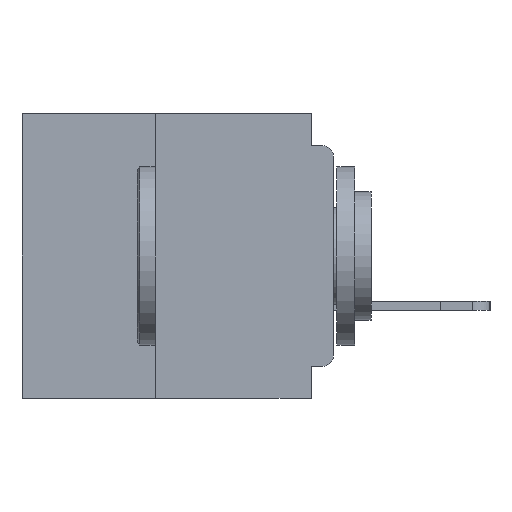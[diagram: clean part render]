
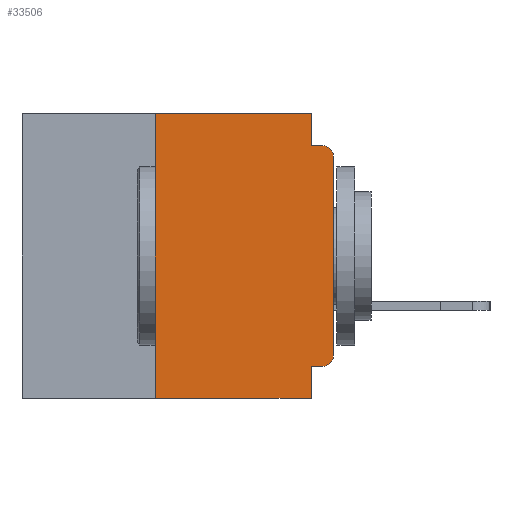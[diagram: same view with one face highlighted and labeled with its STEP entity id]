
A CAD part, left-side view. The second image highlights one B-rep face of the part: STEP entity #33506.
In plain terms, the highlighted planar face has unit normal (-1, 0, 0).
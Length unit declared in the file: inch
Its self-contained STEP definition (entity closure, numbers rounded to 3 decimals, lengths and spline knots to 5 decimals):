
#89 = LINE ( 'NONE', #6230, #43889 ) ;
#749 = EDGE_CURVE ( 'NONE', #41392, #6359, #35364, .T. ) ;
#1302 = VERTEX_POINT ( 'NONE', #23947 ) ;
#1709 = AXIS2_PLACEMENT_3D ( 'NONE', #22011, #51377, #26247 ) ;
#2447 = VECTOR ( 'NONE', #11956, 39.37008 ) ;
#2738 = VECTOR ( 'NONE', #22655, 39.37008 ) ;
#3808 = LINE ( 'NONE', #45752, #2447 ) ;
#4059 = EDGE_CURVE ( 'NONE', #29082, #25901, #21482, .T. ) ;
#4437 = VERTEX_POINT ( 'NONE', #18731 ) ;
#4647 = DIRECTION ( 'NONE',  ( 0., -1., 0. ) ) ;
#5487 = CARTESIAN_POINT ( 'NONE',  ( 0., 0.031, 0. ) ) ;
#6230 = CARTESIAN_POINT ( 'NONE',  ( 0., 0., 0. ) ) ;
#6359 = VERTEX_POINT ( 'NONE', #53056 ) ;
#6812 = LINE ( 'NONE', #17221, #50294 ) ;
#6839 = VERTEX_POINT ( 'NONE', #39576 ) ;
#7388 = DIRECTION ( 'NONE',  ( -1., 0., 0. ) ) ;
#7418 = CARTESIAN_POINT ( 'NONE',  ( 0., 0.015, -0.355 ) ) ;
#7684 = VECTOR ( 'NONE', #35061, 39.37008 ) ;
#9363 = EDGE_CURVE ( 'NONE', #1302, #6359, #6812, .T. ) ;
#10701 = PLANE ( 'NONE',  #41313 ) ;
#11185 = CARTESIAN_POINT ( 'NONE',  ( 0., 0.031, -0.045 ) ) ;
#11956 = DIRECTION ( 'NONE',  ( 0., 1., 0. ) ) ;
#12181 = EDGE_CURVE ( 'NONE', #1302, #47097, #12476, .T. ) ;
#12476 = LINE ( 'NONE', #26227, #33668 ) ;
#12588 = EDGE_CURVE ( 'NONE', #29139, #41392, #3808, .T. ) ;
#12941 = AXIS2_PLACEMENT_3D ( 'NONE', #32714, #7388, #36957 ) ;
#13385 = ORIENTED_EDGE ( 'NONE', *, *, #20022, .T. ) ;
#13660 = LINE ( 'NONE', #45556, #26240 ) ;
#14513 = EDGE_CURVE ( 'NONE', #47097, #6839, #25292, .T. ) ;
#14575 = ORIENTED_EDGE ( 'NONE', *, *, #17854, .F. ) ;
#14943 = CARTESIAN_POINT ( 'NONE',  ( 0., 0.031, -0.4 ) ) ;
#15524 = CARTESIAN_POINT ( 'NONE',  ( 0., 0., -0.06 ) ) ;
#16011 = DIRECTION ( 'NONE',  ( 0., -1., 0. ) ) ;
#17221 = CARTESIAN_POINT ( 'NONE',  ( 0., 0.437, -0.4 ) ) ;
#17854 = EDGE_CURVE ( 'NONE', #6839, #24249, #42747, .T. ) ;
#18723 = CARTESIAN_POINT ( 'NONE',  ( 0., 0.25, 0. ) ) ;
#18731 = CARTESIAN_POINT ( 'NONE',  ( 0., 0., -0.34 ) ) ;
#19205 = DIRECTION ( 'NONE',  ( 0., 0., -1. ) ) ;
#20022 = EDGE_CURVE ( 'NONE', #4437, #29082, #89, .T. ) ;
#21482 = CIRCLE ( 'NONE', #12941, 0.015 ) ;
#22011 = CARTESIAN_POINT ( 'NONE',  ( 0., 0.015, -0.34 ) ) ;
#22655 = DIRECTION ( 'NONE',  ( 0., -1., 0. ) ) ;
#23947 = CARTESIAN_POINT ( 'NONE',  ( 0., 0.25, -0.4 ) ) ;
#24110 = VECTOR ( 'NONE', #31407, 39.37008 ) ;
#24249 = VERTEX_POINT ( 'NONE', #11185 ) ;
#25292 = LINE ( 'NONE', #47868, #2738 ) ;
#25406 = ORIENTED_EDGE ( 'NONE', *, *, #12181, .F. ) ;
#25901 = VERTEX_POINT ( 'NONE', #27492 ) ;
#25913 = ORIENTED_EDGE ( 'NONE', *, *, #12588, .F. ) ;
#26227 = CARTESIAN_POINT ( 'NONE',  ( 0., 0.25, -0.4 ) ) ;
#26240 = VECTOR ( 'NONE', #16011, 39.37008 ) ;
#26247 = DIRECTION ( 'NONE',  ( 0., 0., -1. ) ) ;
#27285 = DIRECTION ( 'NONE',  ( 0., 0., 1. ) ) ;
#27492 = CARTESIAN_POINT ( 'NONE',  ( 0., 0.015, -0.045 ) ) ;
#27789 = ORIENTED_EDGE ( 'NONE', *, *, #4059, .T. ) ;
#29082 = VERTEX_POINT ( 'NONE', #15524 ) ;
#29139 = VERTEX_POINT ( 'NONE', #7418 ) ;
#29578 = FACE_OUTER_BOUND ( 'NONE', #45666, .T. ) ;
#31053 = ORIENTED_EDGE ( 'NONE', *, *, #9363, .T. ) ;
#31407 = DIRECTION ( 'NONE',  ( 0., 0., -1. ) ) ;
#31792 = CARTESIAN_POINT ( 'NONE',  ( 0., 0.437, 0. ) ) ;
#32714 = CARTESIAN_POINT ( 'NONE',  ( 0., 0.015, -0.06 ) ) ;
#33506 = ADVANCED_FACE ( 'NONE', ( #29578 ), #10701, .F. ) ;
#33668 = VECTOR ( 'NONE', #51361, 39.37008 ) ;
#35061 = DIRECTION ( 'NONE',  ( 0., 0., -1. ) ) ;
#35364 = LINE ( 'NONE', #14943, #24110 ) ;
#35473 = ORIENTED_EDGE ( 'NONE', *, *, #47576, .T. ) ;
#35710 = ORIENTED_EDGE ( 'NONE', *, *, #749, .F. ) ;
#36957 = DIRECTION ( 'NONE',  ( 0., 0., -1. ) ) ;
#37351 = CARTESIAN_POINT ( 'NONE',  ( 0., 0.031, -0.355 ) ) ;
#37462 = ORIENTED_EDGE ( 'NONE', *, *, #14513, .F. ) ;
#39576 = CARTESIAN_POINT ( 'NONE',  ( 0., 0.031, 0. ) ) ;
#41242 = ORIENTED_EDGE ( 'NONE', *, *, #52048, .F. ) ;
#41313 = AXIS2_PLACEMENT_3D ( 'NONE', #31792, #44525, #19205 ) ;
#41392 = VERTEX_POINT ( 'NONE', #37351 ) ;
#42747 = LINE ( 'NONE', #5487, #7684 ) ;
#43889 = VECTOR ( 'NONE', #27285, 39.37008 ) ;
#44525 = DIRECTION ( 'NONE',  ( 1., 0., 0. ) ) ;
#45556 = CARTESIAN_POINT ( 'NONE',  ( 0., 0., -0.045 ) ) ;
#45666 = EDGE_LOOP ( 'NONE', ( #13385, #27789, #41242, #14575, #37462, #25406, #31053, #35710, #25913, #35473 ) ) ;
#45752 = CARTESIAN_POINT ( 'NONE',  ( 0., 0., -0.355 ) ) ;
#47097 = VERTEX_POINT ( 'NONE', #18723 ) ;
#47576 = EDGE_CURVE ( 'NONE', #29139, #4437, #48598, .T. ) ;
#47868 = CARTESIAN_POINT ( 'NONE',  ( 0., 0.437, 0. ) ) ;
#48598 = CIRCLE ( 'NONE', #1709, 0.015 ) ;
#50294 = VECTOR ( 'NONE', #4647, 39.37008 ) ;
#51361 = DIRECTION ( 'NONE',  ( 0., 0., 1. ) ) ;
#51377 = DIRECTION ( 'NONE',  ( -1., 0., 0. ) ) ;
#52048 = EDGE_CURVE ( 'NONE', #24249, #25901, #13660, .T. ) ;
#53056 = CARTESIAN_POINT ( 'NONE',  ( 0., 0.031, -0.4 ) ) ;
